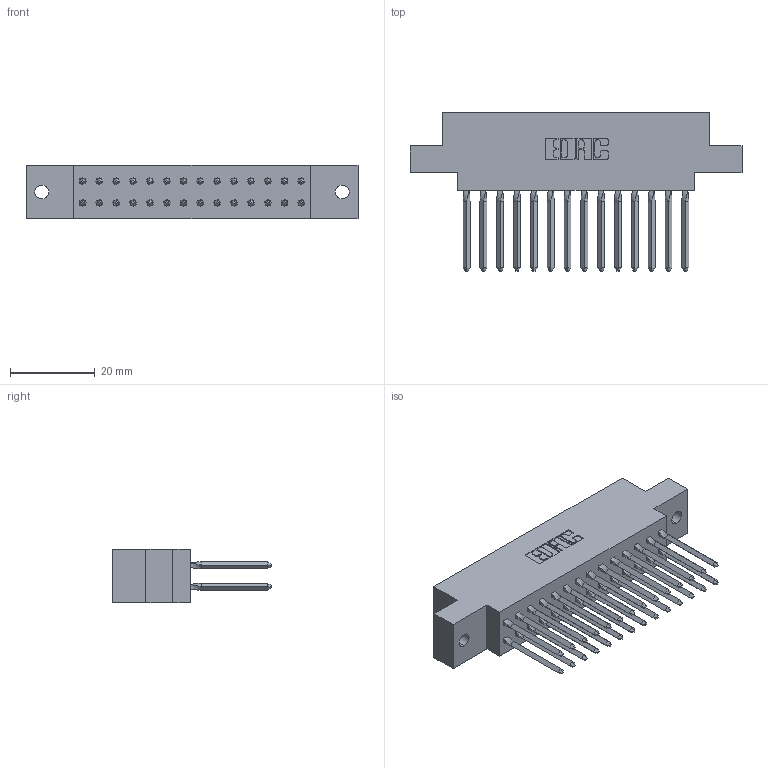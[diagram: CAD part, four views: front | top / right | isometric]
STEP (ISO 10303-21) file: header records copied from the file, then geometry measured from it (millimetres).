
FILE_DESCRIPTION (( 'STEP AP203' ), '1' );
FILE_NAME ('317-028-542-802.STEP', '2020-02-27T19:39:25', ( '' ), ( '' ), 'SwSTEP 2.0', 'SolidWorks 2016', '' );
FILE_SCHEMA (( 'CONFIG_CONTROL_DESIGN' ));
Length unit declared in the file: inch
Products named in the file (3): 317-290-003_542; 317-028-542-802; 317 Part_.144 Dia
Assembly tree (29 placements, depth 2):
  317-028-542-802
    317 Part_.144 Dia
    317-290-003_542  x28
Bounding box: 78.18 x 37.34 x 12.7 mm (x, y, z)
Volume: 11880.4 mm3; surface area: 15356 mm2
Topology: 29 solids, 29 shells, 1698 faces, 4755 edges, 3038 vertices
Faces by surface type: plane 1346, cylinder 240, bspline 112
Entity records: 23163 total; most frequent: CARTESIAN_POINT 4285, ORIENTED_EDGE 3948, DIRECTION 3370, EDGE_CURVE 1974, VECTOR 1804, LINE 1804, VERTEX_POINT 1310, AXIS2_PLACEMENT_3D 783
